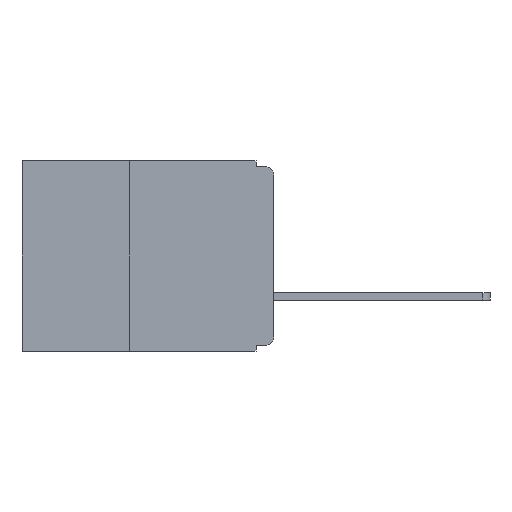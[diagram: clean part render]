
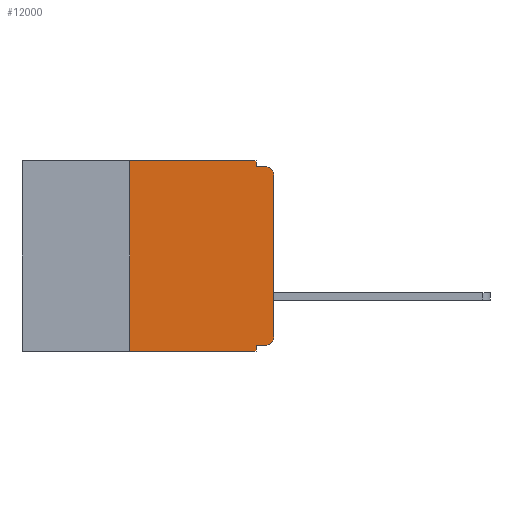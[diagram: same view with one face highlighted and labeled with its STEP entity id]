
A CAD part, left-side view. The second image highlights one B-rep face of the part: STEP entity #12000.
In plain terms, the highlighted planar face has unit normal (-1, 0, 0).
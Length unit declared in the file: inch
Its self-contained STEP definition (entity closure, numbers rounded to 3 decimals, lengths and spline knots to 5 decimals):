
#386 = ORIENTED_EDGE ( 'NONE', *, *, #20144, .T. ) ;
#787 = DIRECTION ( 'NONE',  ( 0., 0., -1. ) ) ;
#816 = DIRECTION ( 'NONE',  ( -1., 0., 0. ) ) ;
#818 = CARTESIAN_POINT ( 'NONE',  ( 0., 0.015, -0.025 ) ) ;
#922 = ORIENTED_EDGE ( 'NONE', *, *, #2546, .T. ) ;
#1197 = CARTESIAN_POINT ( 'NONE',  ( 0., 0.25, 0. ) ) ;
#1210 = CARTESIAN_POINT ( 'NONE',  ( 0., 0.031, 0. ) ) ;
#1323 = CARTESIAN_POINT ( 'NONE',  ( 0., 0.25, -0.33 ) ) ;
#1537 = EDGE_LOOP ( 'NONE', ( #386, #922, #9348, #9825, #13973, #10315, #14452, #10809, #19086, #11297 ) ) ;
#1750 = DIRECTION ( 'NONE',  ( 0., 0., 1. ) ) ;
#1865 = VECTOR ( 'NONE', #15101, 39.37008 ) ;
#2294 = CARTESIAN_POINT ( 'NONE',  ( 0., 0.031, -0.33 ) ) ;
#2464 = CARTESIAN_POINT ( 'NONE',  ( 0., 0.437, -0.33 ) ) ;
#2546 = EDGE_CURVE ( 'NONE', #6869, #16271, #5499, .T. ) ;
#3044 = DIRECTION ( 'NONE',  ( 0., -1., 0. ) ) ;
#3188 = DIRECTION ( 'NONE',  ( -1., 0., 0. ) ) ;
#3201 = VECTOR ( 'NONE', #18094, 39.37008 ) ;
#3277 = AXIS2_PLACEMENT_3D ( 'NONE', #818, #816, #787 ) ;
#3384 = CARTESIAN_POINT ( 'NONE',  ( 0., 0., -0.32 ) ) ;
#3759 = EDGE_CURVE ( 'NONE', #13688, #13164, #12003, .T. ) ;
#4093 = DIRECTION ( 'NONE',  ( 0., -1., 0. ) ) ;
#4146 = CARTESIAN_POINT ( 'NONE',  ( 0., 0., -0.025 ) ) ;
#4376 = VECTOR ( 'NONE', #8921, 39.37008 ) ;
#4560 = CARTESIAN_POINT ( 'NONE',  ( 0., 0.437, 0. ) ) ;
#4868 = LINE ( 'NONE', #13541, #4376 ) ;
#4869 = CARTESIAN_POINT ( 'NONE',  ( 0., 0.031, -0.01 ) ) ;
#5090 = VERTEX_POINT ( 'NONE', #4869 ) ;
#5377 = VERTEX_POINT ( 'NONE', #2294 ) ;
#5499 = CIRCLE ( 'NONE', #3277, 0.015 ) ;
#6430 = LINE ( 'NONE', #9616, #14212 ) ;
#6468 = EDGE_CURVE ( 'NONE', #13164, #9952, #19196, .T. ) ;
#6596 = EDGE_CURVE ( 'NONE', #16483, #8277, #17712, .T. ) ;
#6869 = VERTEX_POINT ( 'NONE', #4146 ) ;
#7162 = CARTESIAN_POINT ( 'NONE',  ( 0., 0., -0.01 ) ) ;
#7444 = LINE ( 'NONE', #7162, #7920 ) ;
#7920 = VECTOR ( 'NONE', #16440, 39.37008 ) ;
#8277 = VERTEX_POINT ( 'NONE', #12336 ) ;
#8381 = CARTESIAN_POINT ( 'NONE',  ( 0., 0.015, -0.32 ) ) ;
#8615 = EDGE_CURVE ( 'NONE', #13688, #5377, #11818, .T. ) ;
#8921 = DIRECTION ( 'NONE',  ( 0., 0., -1. ) ) ;
#9211 = FACE_OUTER_BOUND ( 'NONE', #1537, .T. ) ;
#9348 = ORIENTED_EDGE ( 'NONE', *, *, #19248, .F. ) ;
#9616 = CARTESIAN_POINT ( 'NONE',  ( 0., 0., 0. ) ) ;
#9687 = DIRECTION ( 'NONE',  ( 0., 1., 0. ) ) ;
#9825 = ORIENTED_EDGE ( 'NONE', *, *, #16683, .F. ) ;
#9952 = VERTEX_POINT ( 'NONE', #1210 ) ;
#10315 = ORIENTED_EDGE ( 'NONE', *, *, #3759, .F. ) ;
#10700 = CARTESIAN_POINT ( 'NONE',  ( 0., 0.015, -0.01 ) ) ;
#10758 = PLANE ( 'NONE',  #16871 ) ;
#10809 = ORIENTED_EDGE ( 'NONE', *, *, #16969, .F. ) ;
#10829 = DIRECTION ( 'NONE',  ( 0., 0., -1. ) ) ;
#11297 = ORIENTED_EDGE ( 'NONE', *, *, #11455, .T. ) ;
#11392 = AXIS2_PLACEMENT_3D ( 'NONE', #12546, #3188, #14124 ) ;
#11455 = EDGE_CURVE ( 'NONE', #16483, #15823, #19464, .T. ) ;
#11818 = LINE ( 'NONE', #2464, #19608 ) ;
#12000 = ADVANCED_FACE ( 'NONE', ( #9211 ), #10758, .F. ) ;
#12003 = LINE ( 'NONE', #18076, #3201 ) ;
#12336 = CARTESIAN_POINT ( 'NONE',  ( 0., 0.031, -0.32 ) ) ;
#12546 = CARTESIAN_POINT ( 'NONE',  ( 0., 0.015, -0.305 ) ) ;
#13092 = VECTOR ( 'NONE', #9687, 39.37008 ) ;
#13164 = VERTEX_POINT ( 'NONE', #1197 ) ;
#13541 = CARTESIAN_POINT ( 'NONE',  ( 0., 0.031, -0.33 ) ) ;
#13688 = VERTEX_POINT ( 'NONE', #1323 ) ;
#13973 = ORIENTED_EDGE ( 'NONE', *, *, #6468, .F. ) ;
#14124 = DIRECTION ( 'NONE',  ( 0., 0., -1. ) ) ;
#14212 = VECTOR ( 'NONE', #1750, 39.37008 ) ;
#14384 = LINE ( 'NONE', #19751, #1865 ) ;
#14452 = ORIENTED_EDGE ( 'NONE', *, *, #8615, .T. ) ;
#15040 = VECTOR ( 'NONE', #3044, 39.37008 ) ;
#15101 = DIRECTION ( 'NONE',  ( 0., 0., -1. ) ) ;
#15823 = VERTEX_POINT ( 'NONE', #18962 ) ;
#16271 = VERTEX_POINT ( 'NONE', #10700 ) ;
#16440 = DIRECTION ( 'NONE',  ( 0., -1., 0. ) ) ;
#16483 = VERTEX_POINT ( 'NONE', #8381 ) ;
#16683 = EDGE_CURVE ( 'NONE', #9952, #5090, #14384, .T. ) ;
#16871 = AXIS2_PLACEMENT_3D ( 'NONE', #4560, #20168, #10829 ) ;
#16969 = EDGE_CURVE ( 'NONE', #8277, #5377, #4868, .T. ) ;
#17712 = LINE ( 'NONE', #3384, #13092 ) ;
#18076 = CARTESIAN_POINT ( 'NONE',  ( 0., 0.25, -0.33 ) ) ;
#18094 = DIRECTION ( 'NONE',  ( 0., 0., 1. ) ) ;
#18962 = CARTESIAN_POINT ( 'NONE',  ( 0., 0., -0.305 ) ) ;
#19086 = ORIENTED_EDGE ( 'NONE', *, *, #6596, .F. ) ;
#19196 = LINE ( 'NONE', #20118, #15040 ) ;
#19248 = EDGE_CURVE ( 'NONE', #5090, #16271, #7444, .T. ) ;
#19464 = CIRCLE ( 'NONE', #11392, 0.015 ) ;
#19608 = VECTOR ( 'NONE', #4093, 39.37008 ) ;
#19751 = CARTESIAN_POINT ( 'NONE',  ( 0., 0.031, 0. ) ) ;
#20118 = CARTESIAN_POINT ( 'NONE',  ( 0., 0.437, 0. ) ) ;
#20144 = EDGE_CURVE ( 'NONE', #15823, #6869, #6430, .T. ) ;
#20168 = DIRECTION ( 'NONE',  ( 1., 0., 0. ) ) ;
